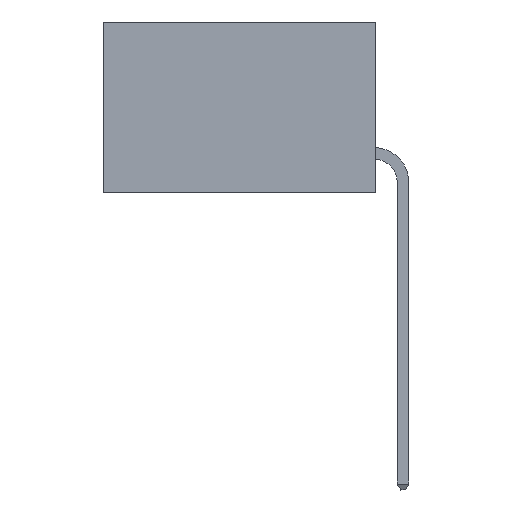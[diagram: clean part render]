
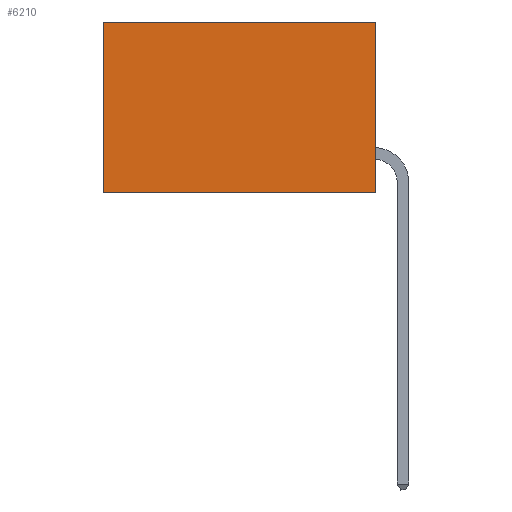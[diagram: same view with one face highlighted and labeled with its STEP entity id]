
A CAD part, left-side view. The second image highlights one B-rep face of the part: STEP entity #6210.
In plain terms, the highlighted planar face has unit normal (-1, 0, 0).
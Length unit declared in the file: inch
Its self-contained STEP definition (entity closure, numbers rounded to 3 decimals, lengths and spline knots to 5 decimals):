
#12 = VECTOR ( 'NONE', #7447, 39.37008 ) ;
#274 = DIRECTION ( 'NONE',  ( 0., 1., 0. ) ) ;
#334 = CARTESIAN_POINT ( 'NONE',  ( 0.277, 0., -0.37 ) ) ;
#687 = VERTEX_POINT ( 'NONE', #3051 ) ;
#1157 = VERTEX_POINT ( 'NONE', #1999 ) ;
#1999 = CARTESIAN_POINT ( 'NONE',  ( 0.277, 0.59, 0. ) ) ;
#2335 = LINE ( 'NONE', #334, #10930 ) ;
#2500 = CARTESIAN_POINT ( 'NONE',  ( 0.277, 0.59, -0.37 ) ) ;
#2801 = ORIENTED_EDGE ( 'NONE', *, *, #15098, .T. ) ;
#3051 = CARTESIAN_POINT ( 'NONE',  ( 0.277, 0., 0. ) ) ;
#3278 = VECTOR ( 'NONE', #7932, 39.37008 ) ;
#6194 = AXIS2_PLACEMENT_3D ( 'NONE', #7191, #7158, #7115 ) ;
#6210 = ADVANCED_FACE ( 'NONE', ( #7913 ), #7205, .F. ) ;
#6734 = CARTESIAN_POINT ( 'NONE',  ( 0.277, 0., -0.37 ) ) ;
#6847 = EDGE_CURVE ( 'NONE', #11427, #13465, #2335, .T. ) ;
#7115 = DIRECTION ( 'NONE',  ( 0., 0., -1. ) ) ;
#7158 = DIRECTION ( 'NONE',  ( 1., 0., 0. ) ) ;
#7191 = CARTESIAN_POINT ( 'NONE',  ( 0.277, 0., -0.37 ) ) ;
#7205 = PLANE ( 'NONE',  #6194 ) ;
#7257 = CARTESIAN_POINT ( 'NONE',  ( 0.277, 0.59, -0.37 ) ) ;
#7447 = DIRECTION ( 'NONE',  ( 0., 0., -1. ) ) ;
#7816 = EDGE_CURVE ( 'NONE', #687, #11427, #9724, .T. ) ;
#7886 = CARTESIAN_POINT ( 'NONE',  ( 0.277, 0., -0.37 ) ) ;
#7897 = ORIENTED_EDGE ( 'NONE', *, *, #7816, .F. ) ;
#7913 = FACE_OUTER_BOUND ( 'NONE', #11798, .T. ) ;
#7932 = DIRECTION ( 'NONE',  ( 0., 0., -1. ) ) ;
#8316 = CARTESIAN_POINT ( 'NONE',  ( 0.277, 0., 0. ) ) ;
#9724 = LINE ( 'NONE', #7886, #3278 ) ;
#9819 = VECTOR ( 'NONE', #10761, 39.37008 ) ;
#10761 = DIRECTION ( 'NONE',  ( 0., 1., 0. ) ) ;
#10930 = VECTOR ( 'NONE', #274, 39.37008 ) ;
#11427 = VERTEX_POINT ( 'NONE', #6734 ) ;
#11798 = EDGE_LOOP ( 'NONE', ( #12518, #14940, #7897, #2801 ) ) ;
#12314 = EDGE_CURVE ( 'NONE', #1157, #13465, #12948, .T. ) ;
#12518 = ORIENTED_EDGE ( 'NONE', *, *, #12314, .T. ) ;
#12948 = LINE ( 'NONE', #2500, #12 ) ;
#13465 = VERTEX_POINT ( 'NONE', #7257 ) ;
#14940 = ORIENTED_EDGE ( 'NONE', *, *, #6847, .F. ) ;
#15098 = EDGE_CURVE ( 'NONE', #687, #1157, #15493, .T. ) ;
#15493 = LINE ( 'NONE', #8316, #9819 ) ;
